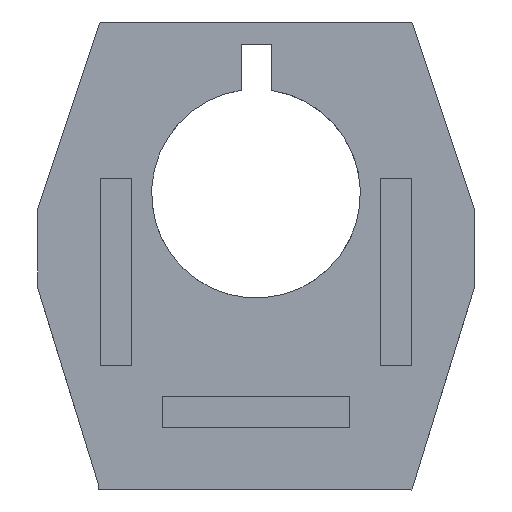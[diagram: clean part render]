
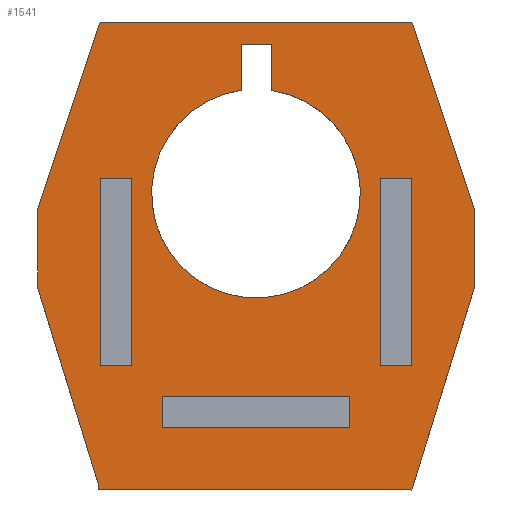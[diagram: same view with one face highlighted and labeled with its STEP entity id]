
A CAD part, front view. The second image highlights one B-rep face of the part: STEP entity #1541.
In plain terms, the highlighted planar face has unit normal (0, -1, 0).
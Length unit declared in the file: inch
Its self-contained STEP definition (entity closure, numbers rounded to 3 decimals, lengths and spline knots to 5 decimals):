
#28=FACE_BOUND('',#169,.T.);
#29=FACE_BOUND('',#170,.T.);
#30=FACE_BOUND('',#171,.T.);
#31=FACE_BOUND('',#172,.T.);
#38=CIRCLE('',#1645,0.33465);
#81=FACE_OUTER_BOUND('',#168,.T.);
#168=EDGE_LOOP('',(#1218,#1219,#1220,#1221,#1222,#1223,#1224,#1225,#1226));
#169=EDGE_LOOP('',(#1227,#1228,#1229,#1230));
#170=EDGE_LOOP('',(#1231,#1232,#1233,#1234));
#171=EDGE_LOOP('',(#1235,#1236,#1237,#1238));
#172=EDGE_LOOP('',(#1239,#1240,#1241,#1242));
#314=LINE('',#2283,#523);
#317=LINE('',#2288,#526);
#320=LINE('',#2296,#529);
#324=LINE('',#2303,#533);
#330=LINE('',#2317,#539);
#333=LINE('',#2322,#542);
#334=LINE('',#2326,#543);
#335=LINE('',#2328,#544);
#336=LINE('',#2330,#545);
#337=LINE('',#2332,#546);
#338=LINE('',#2334,#547);
#339=LINE('',#2336,#548);
#340=LINE('',#2338,#549);
#341=LINE('',#2340,#550);
#342=LINE('',#2341,#551);
#343=LINE('',#2343,#552);
#344=LINE('',#2344,#553);
#345=LINE('',#2346,#554);
#346=LINE('',#2347,#555);
#347=LINE('',#2349,#556);
#348=LINE('',#2350,#557);
#349=LINE('',#2355,#558);
#350=LINE('',#2357,#559);
#351=LINE('',#2358,#560);
#523=VECTOR('',#1866,0.3937);
#526=VECTOR('',#1871,0.3937);
#529=VECTOR('',#1876,0.3937);
#533=VECTOR('',#1882,0.3937);
#539=VECTOR('',#1892,0.3937);
#542=VECTOR('',#1897,0.3937);
#543=VECTOR('',#1900,0.3937);
#544=VECTOR('',#1901,0.3937);
#545=VECTOR('',#1902,0.3937);
#546=VECTOR('',#1903,0.3937);
#547=VECTOR('',#1904,0.3937);
#548=VECTOR('',#1905,0.3937);
#549=VECTOR('',#1906,0.3937);
#550=VECTOR('',#1907,0.3937);
#551=VECTOR('',#1908,0.3937);
#552=VECTOR('',#1909,0.3937);
#553=VECTOR('',#1910,0.3937);
#554=VECTOR('',#1911,0.3937);
#555=VECTOR('',#1912,0.3937);
#556=VECTOR('',#1913,0.3937);
#557=VECTOR('',#1914,0.3937);
#558=VECTOR('',#1917,0.3937);
#559=VECTOR('',#1918,0.3937);
#560=VECTOR('',#1919,0.3937);
#701=VERTEX_POINT('',#2280);
#702=VERTEX_POINT('',#2282);
#703=VERTEX_POINT('',#2286);
#706=VERTEX_POINT('',#2293);
#707=VERTEX_POINT('',#2295);
#709=VERTEX_POINT('',#2301);
#714=VERTEX_POINT('',#2314);
#715=VERTEX_POINT('',#2316);
#716=VERTEX_POINT('',#2320);
#717=VERTEX_POINT('',#2324);
#718=VERTEX_POINT('',#2325);
#719=VERTEX_POINT('',#2327);
#720=VERTEX_POINT('',#2329);
#721=VERTEX_POINT('',#2331);
#722=VERTEX_POINT('',#2333);
#723=VERTEX_POINT('',#2335);
#724=VERTEX_POINT('',#2337);
#725=VERTEX_POINT('',#2339);
#726=VERTEX_POINT('',#2342);
#727=VERTEX_POINT('',#2345);
#728=VERTEX_POINT('',#2348);
#729=VERTEX_POINT('',#2351);
#730=VERTEX_POINT('',#2352);
#731=VERTEX_POINT('',#2354);
#732=VERTEX_POINT('',#2356);
#878=EDGE_CURVE('',#702,#701,#314,.T.);
#881=EDGE_CURVE('',#701,#703,#317,.T.);
#884=EDGE_CURVE('',#707,#706,#320,.T.);
#888=EDGE_CURVE('',#706,#709,#324,.T.);
#894=EDGE_CURVE('',#715,#714,#330,.T.);
#897=EDGE_CURVE('',#714,#716,#333,.T.);
#898=EDGE_CURVE('',#717,#718,#334,.T.);
#899=EDGE_CURVE('',#718,#719,#335,.T.);
#900=EDGE_CURVE('',#719,#720,#336,.T.);
#901=EDGE_CURVE('',#720,#721,#337,.T.);
#902=EDGE_CURVE('',#721,#722,#338,.T.);
#903=EDGE_CURVE('',#722,#723,#339,.T.);
#904=EDGE_CURVE('',#723,#724,#340,.T.);
#905=EDGE_CURVE('',#724,#725,#341,.T.);
#906=EDGE_CURVE('',#725,#717,#342,.T.);
#907=EDGE_CURVE('',#709,#726,#343,.T.);
#908=EDGE_CURVE('',#726,#707,#344,.T.);
#909=EDGE_CURVE('',#703,#727,#345,.T.);
#910=EDGE_CURVE('',#727,#702,#346,.T.);
#911=EDGE_CURVE('',#716,#728,#347,.T.);
#912=EDGE_CURVE('',#728,#715,#348,.T.);
#913=EDGE_CURVE('',#729,#730,#38,.T.);
#914=EDGE_CURVE('',#730,#731,#349,.T.);
#915=EDGE_CURVE('',#731,#732,#350,.T.);
#916=EDGE_CURVE('',#732,#729,#351,.T.);
#1218=ORIENTED_EDGE('',*,*,#898,.T.);
#1219=ORIENTED_EDGE('',*,*,#899,.T.);
#1220=ORIENTED_EDGE('',*,*,#900,.T.);
#1221=ORIENTED_EDGE('',*,*,#901,.T.);
#1222=ORIENTED_EDGE('',*,*,#902,.T.);
#1223=ORIENTED_EDGE('',*,*,#903,.T.);
#1224=ORIENTED_EDGE('',*,*,#904,.T.);
#1225=ORIENTED_EDGE('',*,*,#905,.T.);
#1226=ORIENTED_EDGE('',*,*,#906,.T.);
#1227=ORIENTED_EDGE('',*,*,#907,.T.);
#1228=ORIENTED_EDGE('',*,*,#908,.T.);
#1229=ORIENTED_EDGE('',*,*,#884,.T.);
#1230=ORIENTED_EDGE('',*,*,#888,.T.);
#1231=ORIENTED_EDGE('',*,*,#909,.T.);
#1232=ORIENTED_EDGE('',*,*,#910,.T.);
#1233=ORIENTED_EDGE('',*,*,#878,.T.);
#1234=ORIENTED_EDGE('',*,*,#881,.T.);
#1235=ORIENTED_EDGE('',*,*,#911,.T.);
#1236=ORIENTED_EDGE('',*,*,#912,.T.);
#1237=ORIENTED_EDGE('',*,*,#894,.T.);
#1238=ORIENTED_EDGE('',*,*,#897,.T.);
#1239=ORIENTED_EDGE('',*,*,#913,.T.);
#1240=ORIENTED_EDGE('',*,*,#914,.T.);
#1241=ORIENTED_EDGE('',*,*,#915,.T.);
#1242=ORIENTED_EDGE('',*,*,#916,.T.);
#1460=PLANE('',#1644);
#1541=ADVANCED_FACE('',(#81,#28,#29,#30,#31),#1460,.F.);
#1644=AXIS2_PLACEMENT_3D('',#2323,#1898,#1899);
#1645=AXIS2_PLACEMENT_3D('',#2353,#1915,#1916);
#1866=DIRECTION('',(0.,0.,1.));
#1871=DIRECTION('',(1.,0.,0.));
#1876=DIRECTION('',(0.,0.,1.));
#1882=DIRECTION('',(1.,0.,0.));
#1892=DIRECTION('',(0.,0.,1.));
#1897=DIRECTION('',(1.,0.,0.));
#1898=DIRECTION('center_axis',(0.,1.,0.));
#1899=DIRECTION('ref_axis',(-1.,0.,0.));
#1900=DIRECTION('',(0.294,0.,-0.956));
#1901=DIRECTION('',(0.,0.,-1.));
#1902=DIRECTION('',(1.,0.,0.));
#1903=DIRECTION('',(0.294,0.,0.956));
#1904=DIRECTION('',(0.,0.,1.));
#1905=DIRECTION('',(-0.316,0.,0.949));
#1906=DIRECTION('',(-1.,0.,0.));
#1907=DIRECTION('',(-0.316,0.,-0.949));
#1908=DIRECTION('',(0.,0.,-1.));
#1909=DIRECTION('',(0.,0.,-1.));
#1910=DIRECTION('',(-1.,0.,0.));
#1911=DIRECTION('',(0.,0.,-1.));
#1912=DIRECTION('',(-1.,0.,0.));
#1913=DIRECTION('',(0.,0.,-1.));
#1914=DIRECTION('',(-1.,0.,0.));
#1915=DIRECTION('center_axis',(0.,1.,0.));
#1916=DIRECTION('ref_axis',(-1.,0.,0.));
#1917=DIRECTION('',(0.,0.,1.));
#1918=DIRECTION('',(1.,0.,0.));
#1919=DIRECTION('',(0.,0.,-1.));
#2280=CARTESIAN_POINT('',(-0.3,12.,-0.2));
#2282=CARTESIAN_POINT('',(-0.3,12.,-0.3));
#2283=CARTESIAN_POINT('',(-0.3,12.,-0.025));
#2286=CARTESIAN_POINT('',(0.3,12.,-0.2));
#2288=CARTESIAN_POINT('',(-0.15,12.,-0.2));
#2293=CARTESIAN_POINT('',(-0.5,12.,0.5));
#2295=CARTESIAN_POINT('',(-0.5,12.,-0.1));
#2296=CARTESIAN_POINT('',(-0.5,12.,0.075));
#2301=CARTESIAN_POINT('',(-0.4,12.,0.5));
#2303=CARTESIAN_POINT('',(-0.25,12.,0.5));
#2314=CARTESIAN_POINT('',(0.4,12.,0.5));
#2316=CARTESIAN_POINT('',(0.4,12.,-0.1));
#2317=CARTESIAN_POINT('',(0.4,12.,0.075));
#2320=CARTESIAN_POINT('',(0.5,12.,0.5));
#2322=CARTESIAN_POINT('',(0.2,12.,0.5));
#2323=CARTESIAN_POINT('Origin',(0.,12.,0.25));
#2324=CARTESIAN_POINT('',(-0.7,12.,0.15));
#2325=CARTESIAN_POINT('',(-0.50506,12.,-0.48354));
#2326=CARTESIAN_POINT('',(-0.58378,12.,-0.2277));
#2327=CARTESIAN_POINT('',(-0.50506,12.,-0.5));
#2328=CARTESIAN_POINT('',(-0.50506,12.,0.625));
#2329=CARTESIAN_POINT('',(0.5,12.,-0.5));
#2330=CARTESIAN_POINT('',(-0.2,12.,-0.5));
#2331=CARTESIAN_POINT('',(0.7,12.,0.15));
#2332=CARTESIAN_POINT('',(0.68378,12.,0.0973));
#2333=CARTESIAN_POINT('',(0.7,12.,0.4));
#2334=CARTESIAN_POINT('',(0.7,12.,0.325));
#2335=CARTESIAN_POINT('',(0.5,12.,1.));
#2336=CARTESIAN_POINT('',(0.5875,12.,0.7375));
#2337=CARTESIAN_POINT('',(-0.5,12.,1.));
#2338=CARTESIAN_POINT('',(-0.25,12.,1.));
#2339=CARTESIAN_POINT('',(-0.7,12.,0.4));
#2340=CARTESIAN_POINT('',(-0.6875,12.,0.4375));
#2341=CARTESIAN_POINT('',(-0.7,12.,0.2));
#2342=CARTESIAN_POINT('',(-0.4,12.,-0.1));
#2343=CARTESIAN_POINT('',(-0.4,12.,0.375));
#2344=CARTESIAN_POINT('',(-0.2,12.,-0.1));
#2345=CARTESIAN_POINT('',(0.3,12.,-0.3));
#2346=CARTESIAN_POINT('',(0.3,12.,0.025));
#2347=CARTESIAN_POINT('',(0.15,12.,-0.3));
#2348=CARTESIAN_POINT('',(0.5,12.,-0.1));
#2349=CARTESIAN_POINT('',(0.5,12.,0.375));
#2350=CARTESIAN_POINT('',(0.25,12.,-0.1));
#2351=CARTESIAN_POINT('',(0.05072,12.,0.78078));
#2352=CARTESIAN_POINT('',(-0.0477,12.,0.78123));
#2353=CARTESIAN_POINT('Origin',(0.,12.,0.45));
#2354=CARTESIAN_POINT('',(-0.0477,12.,0.92834));
#2355=CARTESIAN_POINT('',(-0.0477,12.,0.58917));
#2356=CARTESIAN_POINT('',(0.05072,12.,0.92834));
#2357=CARTESIAN_POINT('',(0.02536,12.,0.92834));
#2358=CARTESIAN_POINT('',(0.05072,12.,0.51539));
